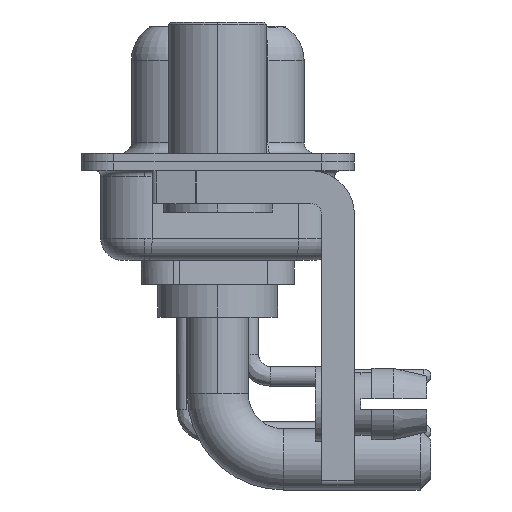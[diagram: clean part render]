
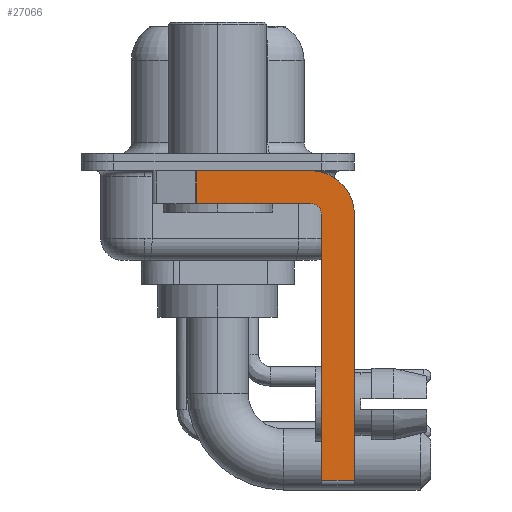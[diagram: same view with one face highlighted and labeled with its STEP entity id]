
A CAD part, left-side view. The second image highlights one B-rep face of the part: STEP entity #27066.
In plain terms, the highlighted planar face has unit normal (-1, 0, 0).
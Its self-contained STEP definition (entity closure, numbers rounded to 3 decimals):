
#1690 = PLANE ( 'NONE',  #17514 ) ;
#2727 = EDGE_CURVE ( 'NONE', #18063, #9614, #22522, .T. ) ;
#3513 = ORIENTED_EDGE ( 'NONE', *, *, #20624, .F. ) ;
#3590 = VERTEX_POINT ( 'NONE', #24744 ) ;
#4022 = DIRECTION ( 'NONE',  ( 0., -1., 0. ) ) ;
#4511 = VECTOR ( 'NONE', #15236, 1000. ) ;
#4606 = ORIENTED_EDGE ( 'NONE', *, *, #2727, .F. ) ;
#4776 = VECTOR ( 'NONE', #9777, 1000. ) ;
#5500 = CIRCLE ( 'NONE', #14809, 2. ) ;
#5841 = CARTESIAN_POINT ( 'NONE',  ( -2.9, -6.25, -14.55 ) ) ;
#7281 = EDGE_CURVE ( 'NONE', #8212, #23056, #25872, .T. ) ;
#7299 = VECTOR ( 'NONE', #7721, 1000. ) ;
#7467 = CARTESIAN_POINT ( 'NONE',  ( -2.9, 0.978, -0.4 ) ) ;
#7721 = DIRECTION ( 'NONE',  ( 0., 1., 0. ) ) ;
#8212 = VERTEX_POINT ( 'NONE', #7467 ) ;
#8973 = CARTESIAN_POINT ( 'NONE',  ( -2.9, -4.25, -1.9 ) ) ;
#8983 = FACE_OUTER_BOUND ( 'NONE', #22996, .T. ) ;
#9614 = VERTEX_POINT ( 'NONE', #5841 ) ;
#9777 = DIRECTION ( 'NONE',  ( 0., 0., -1. ) ) ;
#10130 = EDGE_CURVE ( 'NONE', #8212, #3590, #21464, .T. ) ;
#10428 = ORIENTED_EDGE ( 'NONE', *, *, #23143, .F. ) ;
#11763 = CIRCLE ( 'NONE', #18320, 0.5 ) ;
#11798 = EDGE_CURVE ( 'NONE', #20029, #17417, #11763, .T. ) ;
#11971 = ORIENTED_EDGE ( 'NONE', *, *, #23734, .F. ) ;
#12440 = LINE ( 'NONE', #19162, #22362 ) ;
#13022 = DIRECTION ( 'NONE',  ( 0., 0., 1. ) ) ;
#13081 = CARTESIAN_POINT ( 'NONE',  ( -2.9, -4.25, -2.4 ) ) ;
#13361 = ORIENTED_EDGE ( 'NONE', *, *, #7281, .F. ) ;
#13360 = DIRECTION ( 'NONE',  ( 0., 0., -1. ) ) ;
#13958 = VECTOR ( 'NONE', #4022, 1000. ) ;
#14282 = CARTESIAN_POINT ( 'NONE',  ( -2.9, -4.25, -2.4 ) ) ;
#14809 = AXIS2_PLACEMENT_3D ( 'NONE', #14282, #23665, #18953 ) ;
#15236 = DIRECTION ( 'NONE',  ( 0., -1., 0. ) ) ;
#16058 = LINE ( 'NONE', #22977, #7299 ) ;
#16906 = ORIENTED_EDGE ( 'NONE', *, *, #28308, .T. ) ;
#17118 = CARTESIAN_POINT ( 'NONE',  ( -2.9, -4.75, -14.55 ) ) ;
#17417 = VERTEX_POINT ( 'NONE', #8973 ) ;
#17465 = DIRECTION ( 'NONE',  ( 1., 0., 0. ) ) ;
#17514 = AXIS2_PLACEMENT_3D ( 'NONE', #13081, #17465, #13360 ) ;
#17607 = CARTESIAN_POINT ( 'NONE',  ( -2.9, -4.75, -2.4 ) ) ;
#17729 = CARTESIAN_POINT ( 'NONE',  ( -2.9, -4.25, -14.55 ) ) ;
#17812 = DIRECTION ( 'NONE',  ( 0., 0., -1. ) ) ;
#18063 = VERTEX_POINT ( 'NONE', #20194 ) ;
#18320 = AXIS2_PLACEMENT_3D ( 'NONE', #26927, #25177, #20459 ) ;
#18953 = DIRECTION ( 'NONE',  ( 0., 0., -1. ) ) ;
#19162 = CARTESIAN_POINT ( 'NONE',  ( -2.9, -4.75, -14.8 ) ) ;
#20015 = CARTESIAN_POINT ( 'NONE',  ( -2.9, -6.25, -2.4 ) ) ;
#20029 = VERTEX_POINT ( 'NONE', #17607 ) ;
#20194 = CARTESIAN_POINT ( 'NONE',  ( -2.9, -6.25, -2.4 ) ) ;
#20459 = DIRECTION ( 'NONE',  ( 0., 0., 1. ) ) ;
#20624 = EDGE_CURVE ( 'NONE', #17417, #3590, #16058, .T. ) ;
#21464 = LINE ( 'NONE', #25463, #4776 ) ;
#21882 = CARTESIAN_POINT ( 'NONE',  ( -2.9, 3., -0.4 ) ) ;
#22029 = ORIENTED_EDGE ( 'NONE', *, *, #10130, .T. ) ;
#22362 = VECTOR ( 'NONE', #13022, 1000. ) ;
#22522 = LINE ( 'NONE', #20015, #23507 ) ;
#22977 = CARTESIAN_POINT ( 'NONE',  ( -2.9, -4.25, -1.9 ) ) ;
#22996 = EDGE_LOOP ( 'NONE', ( #13361, #22029, #3513, #25335, #11971, #16906, #4606, #10428 ) ) ;
#23056 = VERTEX_POINT ( 'NONE', #27062 ) ;
#23143 = EDGE_CURVE ( 'NONE', #23056, #18063, #5500, .T. ) ;
#23507 = VECTOR ( 'NONE', #17812, 1000. ) ;
#23665 = DIRECTION ( 'NONE',  ( 1., 0., 0. ) ) ;
#23734 = EDGE_CURVE ( 'NONE', #28709, #20029, #12440, .T. ) ;
#24744 = CARTESIAN_POINT ( 'NONE',  ( -2.9, 0.978, -1.9 ) ) ;
#25177 = DIRECTION ( 'NONE',  ( -1., 0., 0. ) ) ;
#25335 = ORIENTED_EDGE ( 'NONE', *, *, #11798, .F. ) ;
#25463 = CARTESIAN_POINT ( 'NONE',  ( -2.9, 0.978, -1.9 ) ) ;
#25872 = LINE ( 'NONE', #21882, #13958 ) ;
#26833 = LINE ( 'NONE', #17729, #4511 ) ;
#26927 = CARTESIAN_POINT ( 'NONE',  ( -2.9, -4.25, -2.4 ) ) ;
#27062 = CARTESIAN_POINT ( 'NONE',  ( -2.9, -4.25, -0.4 ) ) ;
#27066 = ADVANCED_FACE ( 'NONE', ( #8983 ), #1690, .F. ) ;
#28308 = EDGE_CURVE ( 'NONE', #28709, #9614, #26833, .T. ) ;
#28709 = VERTEX_POINT ( 'NONE', #17118 ) ;
